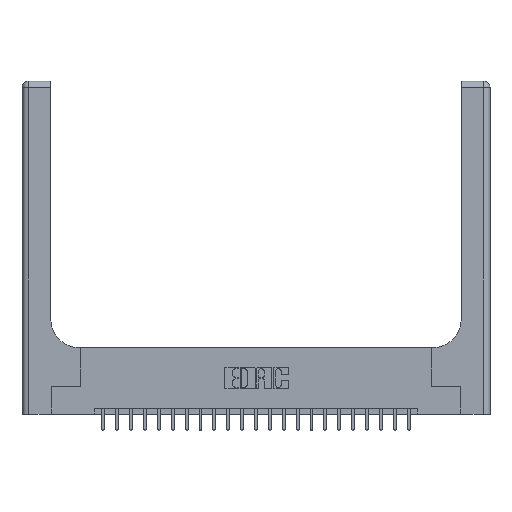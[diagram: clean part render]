
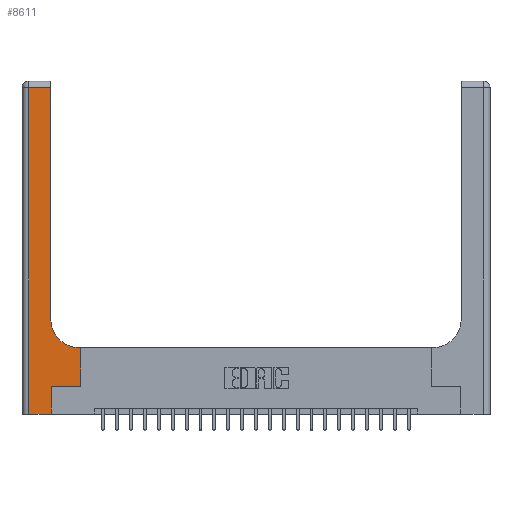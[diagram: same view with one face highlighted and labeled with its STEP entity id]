
A CAD part, top view. The second image highlights one B-rep face of the part: STEP entity #8611.
In plain terms, the highlighted planar face has unit normal (0, 0, 1).
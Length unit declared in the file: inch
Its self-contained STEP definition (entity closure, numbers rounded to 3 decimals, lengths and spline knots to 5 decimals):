
#79 = EDGE_CURVE ( 'NONE', #3897, #15797, #14820, .T. ) ;
#956 = CARTESIAN_POINT ( 'NONE',  ( 0.06, 3., 0.37 ) ) ;
#1047 = CARTESIAN_POINT ( 'NONE',  ( 0.51, 0.6, 0.37 ) ) ;
#1123 = DIRECTION ( 'NONE',  ( 0., -1., 0. ) ) ;
#1407 = VERTEX_POINT ( 'NONE', #18797 ) ;
#1526 = CARTESIAN_POINT ( 'NONE',  ( 0.265, 0.25, 0.37 ) ) ;
#2448 = CARTESIAN_POINT ( 'NONE',  ( 0.06, 0., 0.37 ) ) ;
#3010 = FACE_OUTER_BOUND ( 'NONE', #18895, .T. ) ;
#3897 = VERTEX_POINT ( 'NONE', #2448 ) ;
#4755 = CARTESIAN_POINT ( 'NONE',  ( 0.26, 0.6, 0.37 ) ) ;
#5277 = VERTEX_POINT ( 'NONE', #16315 ) ;
#5357 = LINE ( 'NONE', #17831, #18825 ) ;
#6047 = DIRECTION ( 'NONE',  ( 0., 0., -1. ) ) ;
#6943 = LINE ( 'NONE', #13734, #13809 ) ;
#7184 = LINE ( 'NONE', #18142, #13491 ) ;
#8084 = VERTEX_POINT ( 'NONE', #21994 ) ;
#8324 = ORIENTED_EDGE ( 'NONE', *, *, #8460, .T. ) ;
#8370 = VECTOR ( 'NONE', #1123, 39.37008 ) ;
#8460 = EDGE_CURVE ( 'NONE', #8816, #5277, #7184, .T. ) ;
#8611 = ADVANCED_FACE ( 'NONE', ( #3010 ), #16733, .F. ) ;
#8764 = ORIENTED_EDGE ( 'NONE', *, *, #79, .T. ) ;
#8816 = VERTEX_POINT ( 'NONE', #17366 ) ;
#9008 = ORIENTED_EDGE ( 'NONE', *, *, #21856, .T. ) ;
#9209 = DIRECTION ( 'NONE',  ( 0., 1., 0. ) ) ;
#9475 = DIRECTION ( 'NONE',  ( 0., 0., -1. ) ) ;
#9635 = CARTESIAN_POINT ( 'NONE',  ( 0., 3., 0.37 ) ) ;
#9799 = VERTEX_POINT ( 'NONE', #1047 ) ;
#10064 = VERTEX_POINT ( 'NONE', #19213 ) ;
#10415 = DIRECTION ( 'NONE',  ( 0., 1., 0. ) ) ;
#10451 = AXIS2_PLACEMENT_3D ( 'NONE', #9635, #6047, #21966 ) ;
#10477 = DIRECTION ( 'NONE',  ( 1., 0., 0. ) ) ;
#11120 = ORIENTED_EDGE ( 'NONE', *, *, #13549, .T. ) ;
#11132 = VECTOR ( 'NONE', #20714, 39.37008 ) ;
#11445 = AXIS2_PLACEMENT_3D ( 'NONE', #19724, #9475, #16495 ) ;
#11488 = DIRECTION ( 'NONE',  ( -1., 0., 0. ) ) ;
#12538 = EDGE_CURVE ( 'NONE', #10064, #9799, #18319, .T. ) ;
#12740 = VECTOR ( 'NONE', #11488, 39.37008 ) ;
#13169 = VECTOR ( 'NONE', #10477, 39.37008 ) ;
#13237 = ORIENTED_EDGE ( 'NONE', *, *, #12538, .T. ) ;
#13454 = ORIENTED_EDGE ( 'NONE', *, *, #16642, .T. ) ;
#13491 = VECTOR ( 'NONE', #9209, 39.37008 ) ;
#13549 = EDGE_CURVE ( 'NONE', #1407, #3897, #21835, .T. ) ;
#13734 = CARTESIAN_POINT ( 'NONE',  ( 0.528, 0.25, 0.37 ) ) ;
#13791 = EDGE_CURVE ( 'NONE', #15797, #8084, #5357, .T. ) ;
#13809 = VECTOR ( 'NONE', #10415, 39.37008 ) ;
#13830 = CIRCLE ( 'NONE', #11445, 0.25 ) ;
#14820 = LINE ( 'NONE', #20952, #13169 ) ;
#15179 = ORIENTED_EDGE ( 'NONE', *, *, #13791, .T. ) ;
#15698 = VECTOR ( 'NONE', #17407, 39.37008 ) ;
#15797 = VERTEX_POINT ( 'NONE', #17225 ) ;
#15799 = DIRECTION ( 'NONE',  ( 0., 1., 0. ) ) ;
#16005 = EDGE_CURVE ( 'NONE', #9799, #8816, #13830, .T. ) ;
#16315 = CARTESIAN_POINT ( 'NONE',  ( 0.26, 2.94, 0.37 ) ) ;
#16495 = DIRECTION ( 'NONE',  ( 1., 0., 0. ) ) ;
#16642 = EDGE_CURVE ( 'NONE', #17422, #10064, #6943, .T. ) ;
#16733 = PLANE ( 'NONE',  #10451 ) ;
#17225 = CARTESIAN_POINT ( 'NONE',  ( 0.265, 0., 0.37 ) ) ;
#17366 = CARTESIAN_POINT ( 'NONE',  ( 0.26, 0.85, 0.37 ) ) ;
#17407 = DIRECTION ( 'NONE',  ( 1., 0., 0. ) ) ;
#17422 = VERTEX_POINT ( 'NONE', #21000 ) ;
#17695 = EDGE_CURVE ( 'NONE', #8084, #17422, #21761, .T. ) ;
#17831 = CARTESIAN_POINT ( 'NONE',  ( 0.265, 0., 0.37 ) ) ;
#18142 = CARTESIAN_POINT ( 'NONE',  ( 0.26, 3., 0.37 ) ) ;
#18319 = LINE ( 'NONE', #4755, #11132 ) ;
#18797 = CARTESIAN_POINT ( 'NONE',  ( 0.06, 2.94, 0.37 ) ) ;
#18825 = VECTOR ( 'NONE', #15799, 39.37008 ) ;
#18895 = EDGE_LOOP ( 'NONE', ( #8324, #9008, #11120, #8764, #15179, #21375, #13454, #13237, #22729 ) ) ;
#19213 = CARTESIAN_POINT ( 'NONE',  ( 0.528, 0.6, 0.37 ) ) ;
#19724 = CARTESIAN_POINT ( 'NONE',  ( 0.51, 0.85, 0.37 ) ) ;
#20714 = DIRECTION ( 'NONE',  ( -1., 0., 0. ) ) ;
#20952 = CARTESIAN_POINT ( 'NONE',  ( 0., 0., 0.37 ) ) ;
#21000 = CARTESIAN_POINT ( 'NONE',  ( 0.528, 0.25, 0.37 ) ) ;
#21375 = ORIENTED_EDGE ( 'NONE', *, *, #17695, .T. ) ;
#21761 = LINE ( 'NONE', #1526, #15698 ) ;
#21835 = LINE ( 'NONE', #956, #8370 ) ;
#21856 = EDGE_CURVE ( 'NONE', #5277, #1407, #22106, .T. ) ;
#21887 = CARTESIAN_POINT ( 'NONE',  ( 0., 2.94, 0.37 ) ) ;
#21966 = DIRECTION ( 'NONE',  ( -1., 0., 0. ) ) ;
#21994 = CARTESIAN_POINT ( 'NONE',  ( 0.265, 0.25, 0.37 ) ) ;
#22106 = LINE ( 'NONE', #21887, #12740 ) ;
#22729 = ORIENTED_EDGE ( 'NONE', *, *, #16005, .T. ) ;
